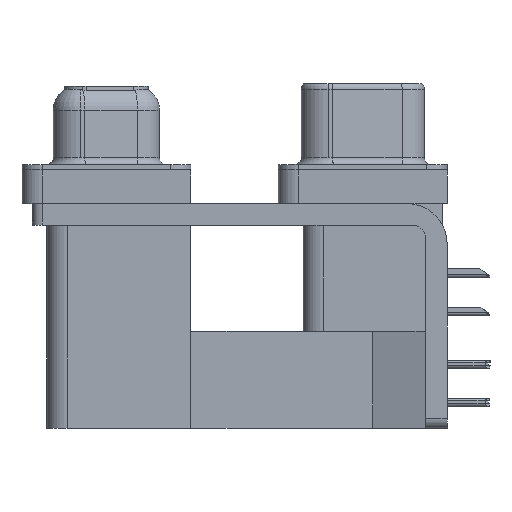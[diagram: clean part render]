
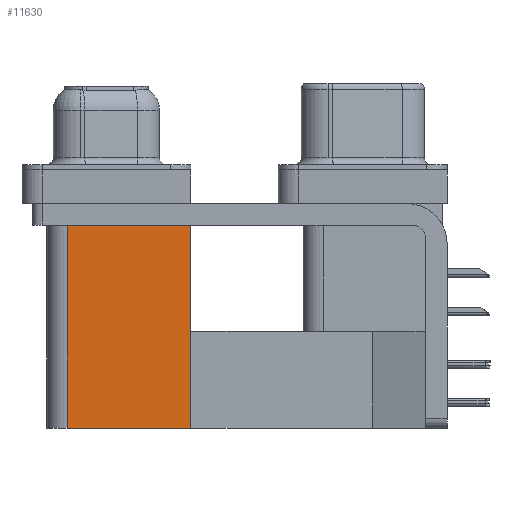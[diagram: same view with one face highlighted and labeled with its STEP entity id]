
A CAD part, left-side view. The second image highlights one B-rep face of the part: STEP entity #11630.
In plain terms, the highlighted planar face has unit normal (-1, 0, 0).
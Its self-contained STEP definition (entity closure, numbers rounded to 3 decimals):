
#1559 = FACE_OUTER_BOUND ( 'NONE', #15873, .T. ) ;
#2961 = LINE ( 'NONE', #5043, #31598 ) ;
#4837 = VERTEX_POINT ( 'NONE', #10025 ) ;
#5043 = CARTESIAN_POINT ( 'NONE',  ( 3.79, 12.775, -19.2 ) ) ;
#5338 = ORIENTED_EDGE ( 'NONE', *, *, #16685, .F. ) ;
#6552 = LINE ( 'NONE', #23870, #10047 ) ;
#7477 = CARTESIAN_POINT ( 'NONE',  ( 3.79, 12.775, -2.5 ) ) ;
#7924 = VERTEX_POINT ( 'NONE', #27613 ) ;
#8250 = ORIENTED_EDGE ( 'NONE', *, *, #31671, .T. ) ;
#9004 = DIRECTION ( 'NONE',  ( 0., 0., 1. ) ) ;
#10025 = CARTESIAN_POINT ( 'NONE',  ( 3.79, 21.975, -19.2 ) ) ;
#10047 = VECTOR ( 'NONE', #18017, 1000. ) ;
#11630 = ADVANCED_FACE ( 'NONE', ( #1559 ), #27370, .F. ) ;
#12370 = LINE ( 'NONE', #32546, #37244 ) ;
#14442 = DIRECTION ( 'NONE',  ( 0., 1., 0. ) ) ;
#15873 = EDGE_LOOP ( 'NONE', ( #8250, #5338, #29639, #22955 ) ) ;
#15902 = AXIS2_PLACEMENT_3D ( 'NONE', #33605, #33975, #33792 ) ;
#16685 = EDGE_CURVE ( 'NONE', #4837, #20533, #6552, .T. ) ;
#18017 = DIRECTION ( 'NONE',  ( 0., 0., 1. ) ) ;
#20533 = VERTEX_POINT ( 'NONE', #27436 ) ;
#22955 = ORIENTED_EDGE ( 'NONE', *, *, #30229, .T. ) ;
#23870 = CARTESIAN_POINT ( 'NONE',  ( 3.79, 21.975, -19.2 ) ) ;
#26198 = EDGE_CURVE ( 'NONE', #29090, #4837, #2961, .T. ) ;
#27370 = PLANE ( 'NONE',  #15902 ) ;
#27436 = CARTESIAN_POINT ( 'NONE',  ( 3.79, 21.975, -2.5 ) ) ;
#27613 = CARTESIAN_POINT ( 'NONE',  ( 3.79, 12.775, -2.5 ) ) ;
#27830 = DIRECTION ( 'NONE',  ( 0., 1., 0. ) ) ;
#29090 = VERTEX_POINT ( 'NONE', #36365 ) ;
#29639 = ORIENTED_EDGE ( 'NONE', *, *, #26198, .F. ) ;
#29664 = VECTOR ( 'NONE', #27830, 1000. ) ;
#30229 = EDGE_CURVE ( 'NONE', #29090, #7924, #12370, .T. ) ;
#31598 = VECTOR ( 'NONE', #14442, 1000. ) ;
#31671 = EDGE_CURVE ( 'NONE', #7924, #20533, #36333, .T. ) ;
#32546 = CARTESIAN_POINT ( 'NONE',  ( 3.79, 12.775, -19.2 ) ) ;
#33605 = CARTESIAN_POINT ( 'NONE',  ( 3.79, 12.775, -19.2 ) ) ;
#33792 = DIRECTION ( 'NONE',  ( 0., 1., 0. ) ) ;
#33975 = DIRECTION ( 'NONE',  ( 1., 0., 0. ) ) ;
#36333 = LINE ( 'NONE', #7477, #29664 ) ;
#36365 = CARTESIAN_POINT ( 'NONE',  ( 3.79, 12.775, -19.2 ) ) ;
#37244 = VECTOR ( 'NONE', #9004, 1000. ) ;
